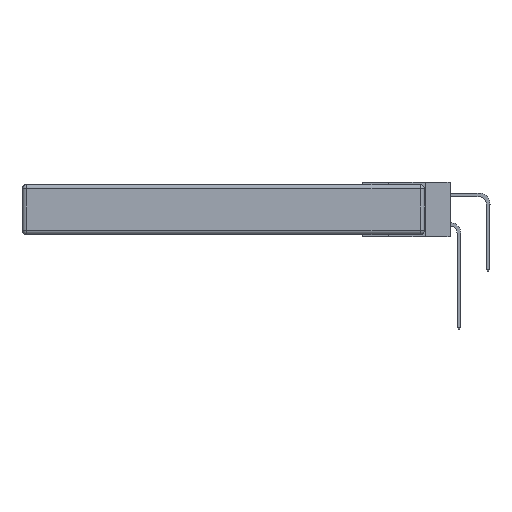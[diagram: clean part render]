
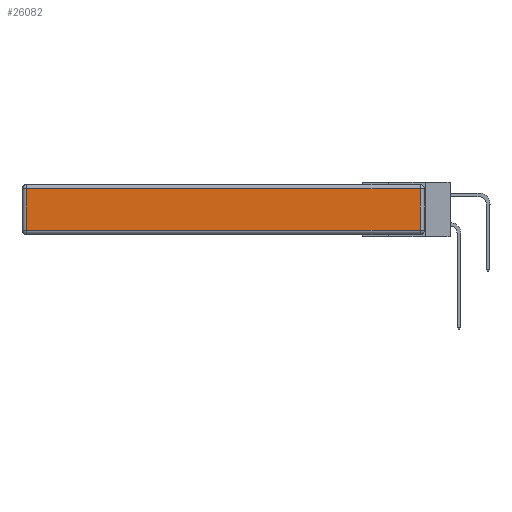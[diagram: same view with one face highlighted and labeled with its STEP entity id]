
A CAD part, left-side view. The second image highlights one B-rep face of the part: STEP entity #26082.
In plain terms, the highlighted planar face has unit normal (-1, 0, 0).
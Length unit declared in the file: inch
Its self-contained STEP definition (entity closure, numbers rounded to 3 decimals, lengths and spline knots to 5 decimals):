
#1196 = VERTEX_POINT ( 'NONE', #2702 ) ;
#1680 = CARTESIAN_POINT ( 'NONE',  ( 0., 2.75, -0.03 ) ) ;
#2283 = DIRECTION ( 'NONE',  ( 0., 0., 1. ) ) ;
#2702 = CARTESIAN_POINT ( 'NONE',  ( 0., 0.03, -0.313 ) ) ;
#5192 = EDGE_CURVE ( 'NONE', #5264, #1196, #8053, .T. ) ;
#5264 = VERTEX_POINT ( 'NONE', #18135 ) ;
#5743 = LINE ( 'NONE', #35274, #11285 ) ;
#7164 = VECTOR ( 'NONE', #29278, 39.37008 ) ;
#7986 = VECTOR ( 'NONE', #12409, 39.37008 ) ;
#8053 = LINE ( 'NONE', #26187, #7164 ) ;
#10823 = DIRECTION ( 'NONE',  ( 0., 0., -1. ) ) ;
#11247 = VERTEX_POINT ( 'NONE', #14080 ) ;
#11285 = VECTOR ( 'NONE', #10823, 39.37008 ) ;
#12409 = DIRECTION ( 'NONE',  ( 0., 1., 0. ) ) ;
#14080 = CARTESIAN_POINT ( 'NONE',  ( 0., 2.72, -0.03 ) ) ;
#15630 = CARTESIAN_POINT ( 'NONE',  ( 0., 0., -0.343 ) ) ;
#16095 = ORIENTED_EDGE ( 'NONE', *, *, #23972, .T. ) ;
#16568 = LINE ( 'NONE', #17119, #28153 ) ;
#17119 = CARTESIAN_POINT ( 'NONE',  ( 0., 0.03, -0.343 ) ) ;
#17885 = ORIENTED_EDGE ( 'NONE', *, *, #28610, .T. ) ;
#18135 = CARTESIAN_POINT ( 'NONE',  ( 0., 2.72, -0.313 ) ) ;
#20228 = AXIS2_PLACEMENT_3D ( 'NONE', #15630, #29272, #2283 ) ;
#20985 = FACE_OUTER_BOUND ( 'NONE', #28667, .T. ) ;
#21731 = EDGE_CURVE ( 'NONE', #1196, #27311, #16568, .T. ) ;
#23972 = EDGE_CURVE ( 'NONE', #11247, #5264, #5743, .T. ) ;
#26082 = ADVANCED_FACE ( 'NONE', ( #20985 ), #29643, .T. ) ;
#26151 = CARTESIAN_POINT ( 'NONE',  ( 0., 0.03, -0.03 ) ) ;
#26168 = ORIENTED_EDGE ( 'NONE', *, *, #5192, .T. ) ;
#26187 = CARTESIAN_POINT ( 'NONE',  ( 0., 0., -0.313 ) ) ;
#27311 = VERTEX_POINT ( 'NONE', #26151 ) ;
#28153 = VECTOR ( 'NONE', #33713, 39.37008 ) ;
#28610 = EDGE_CURVE ( 'NONE', #27311, #11247, #33172, .T. ) ;
#28667 = EDGE_LOOP ( 'NONE', ( #26168, #31562, #17885, #16095 ) ) ;
#29272 = DIRECTION ( 'NONE',  ( -1., 0., 0. ) ) ;
#29278 = DIRECTION ( 'NONE',  ( 0., -1., 0. ) ) ;
#29643 = PLANE ( 'NONE',  #20228 ) ;
#31562 = ORIENTED_EDGE ( 'NONE', *, *, #21731, .T. ) ;
#33172 = LINE ( 'NONE', #1680, #7986 ) ;
#33713 = DIRECTION ( 'NONE',  ( 0., 0., 1. ) ) ;
#35274 = CARTESIAN_POINT ( 'NONE',  ( 0., 2.72, -0.343 ) ) ;
